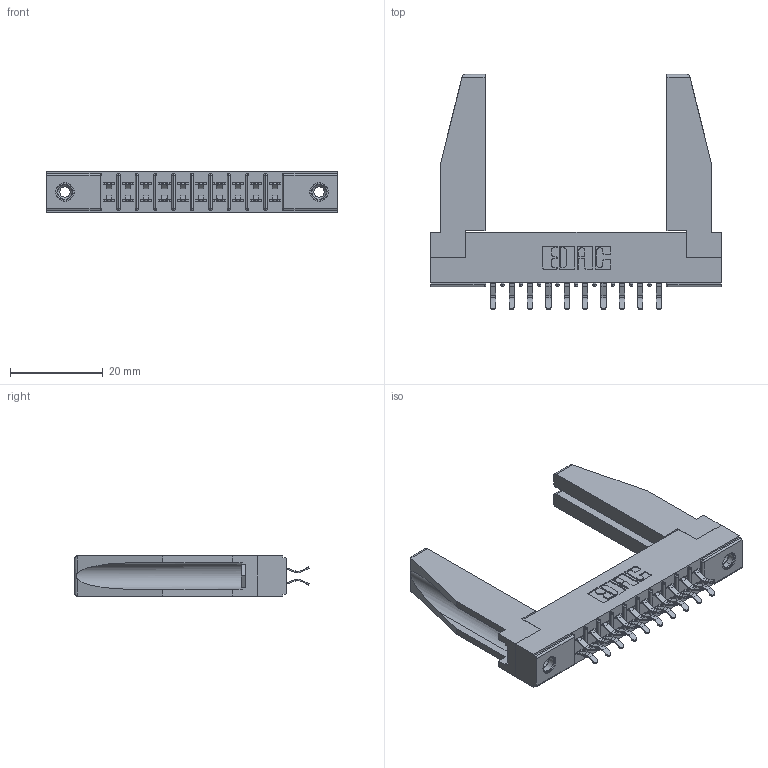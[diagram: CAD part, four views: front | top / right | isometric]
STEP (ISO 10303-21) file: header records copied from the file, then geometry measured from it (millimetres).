
FILE_DESCRIPTION (( 'STEP AP203' ), '1' );
FILE_NAME ('355-020-556-578.STEP', '2019-09-11T03:45:52', ( '' ), ( '' ), 'SwSTEP 2.0', 'SolidWorks 2016', '' );
FILE_SCHEMA (( 'CONFIG_CONTROL_DESIGN' ));
Length unit declared in the file: inch
Products named in the file (5): 305-290-001_556; 355-020-556-578; 305 Part_.156 Dia; 345-250-001_345-250-001-102; 307-220-078
Assembly tree (25 placements, depth 2):
  355-020-556-578
    305 Part_.156 Dia
    305-290-001_556  x20
    345-250-001_345-250-001-102  x2
    307-220-078  x2
Bounding box: 62.64 x 50.67 x 8.71 mm (x, y, z)
Volume: 7791.1 mm3; surface area: 10628.7 mm2
Topology: 25 solids, 25 shells, 1366 faces, 3876 edges, 2520 vertices
Faces by surface type: plane 772, cylinder 538, sphere 40, cone 12, torus 4
Entity records: 17384 total; most frequent: CARTESIAN_POINT 2886, ORIENTED_EDGE 2818, DIRECTION 2779, EDGE_CURVE 1409, LINE 1097, VECTOR 1097, VERTEX_POINT 906, AXIS2_PLACEMENT_3D 841
